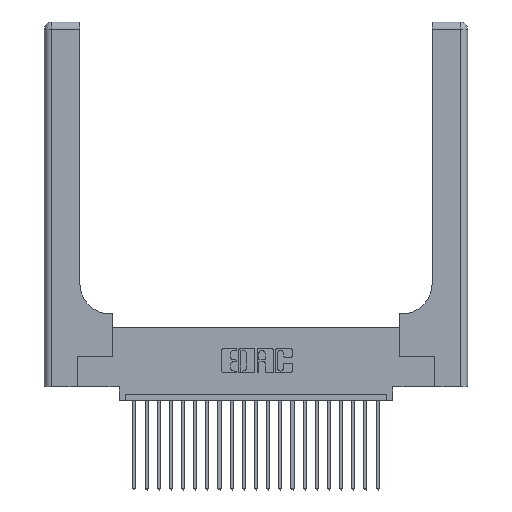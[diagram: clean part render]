
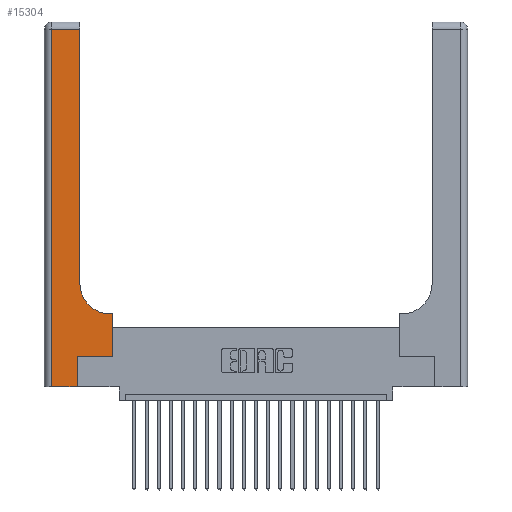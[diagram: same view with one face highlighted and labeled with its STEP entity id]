
A CAD part, top view. The second image highlights one B-rep face of the part: STEP entity #15304.
In plain terms, the highlighted planar face has unit normal (0, 0, 1).
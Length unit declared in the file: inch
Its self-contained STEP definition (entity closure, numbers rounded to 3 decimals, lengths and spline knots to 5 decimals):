
#93 = EDGE_CURVE ( 'NONE', #22028, #8500, #17135, .T. ) ;
#555 = VERTEX_POINT ( 'NONE', #14557 ) ;
#794 = DIRECTION ( 'NONE',  ( 1., 0., 0. ) ) ;
#958 = EDGE_CURVE ( 'NONE', #9788, #2808, #7204, .T. ) ;
#1011 = DIRECTION ( 'NONE',  ( -1., 0., 0. ) ) ;
#2621 = CARTESIAN_POINT ( 'NONE',  ( 0.2915, 3., 0.37 ) ) ;
#2646 = CARTESIAN_POINT ( 'NONE',  ( 0.269, 0., 0.37 ) ) ;
#2687 = EDGE_CURVE ( 'NONE', #6200, #15334, #2757, .T. ) ;
#2757 = LINE ( 'NONE', #19590, #21880 ) ;
#2808 = VERTEX_POINT ( 'NONE', #17730 ) ;
#2962 = LINE ( 'NONE', #18413, #11692 ) ;
#3296 = EDGE_CURVE ( 'NONE', #3470, #6200, #6463, .T. ) ;
#3470 = VERTEX_POINT ( 'NONE', #16917 ) ;
#3796 = EDGE_CURVE ( 'NONE', #8500, #555, #2962, .T. ) ;
#4652 = CARTESIAN_POINT ( 'NONE',  ( 0., 3., 0.37 ) ) ;
#4684 = DIRECTION ( 'NONE',  ( 0., 1., 0. ) ) ;
#4920 = LINE ( 'NONE', #6509, #10421 ) ;
#5051 = DIRECTION ( 'NONE',  ( 0., 1., 0. ) ) ;
#5177 = DIRECTION ( 'NONE',  ( 1., 0., 0. ) ) ;
#5511 = ORIENTED_EDGE ( 'NONE', *, *, #3296, .T. ) ;
#6200 = VERTEX_POINT ( 'NONE', #8472 ) ;
#6463 = LINE ( 'NONE', #14216, #7358 ) ;
#6509 = CARTESIAN_POINT ( 'NONE',  ( 0., 2.94, 0.37 ) ) ;
#6706 = CARTESIAN_POINT ( 'NONE',  ( 0.269, 0.25, 0.37 ) ) ;
#7204 = LINE ( 'NONE', #2621, #10124 ) ;
#7358 = VECTOR ( 'NONE', #5051, 39.37008 ) ;
#8363 = CARTESIAN_POINT ( 'NONE',  ( 0.5415, 0.6, 0.37 ) ) ;
#8472 = CARTESIAN_POINT ( 'NONE',  ( 0.5585, 0.6, 0.37 ) ) ;
#8500 = VERTEX_POINT ( 'NONE', #18981 ) ;
#9495 = CARTESIAN_POINT ( 'NONE',  ( 0.06, 2.94, 0.37 ) ) ;
#9610 = LINE ( 'NONE', #2646, #19750 ) ;
#9763 = ORIENTED_EDGE ( 'NONE', *, *, #3796, .T. ) ;
#9788 = VERTEX_POINT ( 'NONE', #20471 ) ;
#10089 = ORIENTED_EDGE ( 'NONE', *, *, #958, .T. ) ;
#10124 = VECTOR ( 'NONE', #21164, 39.37008 ) ;
#10263 = CARTESIAN_POINT ( 'NONE',  ( 0.06, 3., 0.37 ) ) ;
#10346 = DIRECTION ( 'NONE',  ( 0., -1., 0. ) ) ;
#10421 = VECTOR ( 'NONE', #1011, 39.37008 ) ;
#11050 = EDGE_CURVE ( 'NONE', #15334, #9788, #11296, .T. ) ;
#11296 = CIRCLE ( 'NONE', #23469, 0.25 ) ;
#11692 = VECTOR ( 'NONE', #15731, 39.37008 ) ;
#11892 = DIRECTION ( 'NONE',  ( 0., 0., -1. ) ) ;
#11923 = FACE_OUTER_BOUND ( 'NONE', #21212, .T. ) ;
#12024 = DIRECTION ( 'NONE',  ( -1., 0., 0. ) ) ;
#12341 = VERTEX_POINT ( 'NONE', #6706 ) ;
#12382 = ORIENTED_EDGE ( 'NONE', *, *, #16177, .T. ) ;
#13208 = EDGE_CURVE ( 'NONE', #12341, #3470, #19015, .T. ) ;
#13947 = ORIENTED_EDGE ( 'NONE', *, *, #93, .T. ) ;
#14211 = DIRECTION ( 'NONE',  ( 0., 0., -1. ) ) ;
#14216 = CARTESIAN_POINT ( 'NONE',  ( 0.5585, 0.25, 0.37 ) ) ;
#14430 = ORIENTED_EDGE ( 'NONE', *, *, #11050, .T. ) ;
#14502 = DIRECTION ( 'NONE',  ( -1., 0., 0. ) ) ;
#14557 = CARTESIAN_POINT ( 'NONE',  ( 0.269, 0., 0.37 ) ) ;
#15087 = EDGE_CURVE ( 'NONE', #555, #12341, #9610, .T. ) ;
#15304 = ADVANCED_FACE ( 'NONE', ( #11923 ), #23410, .F. ) ;
#15334 = VERTEX_POINT ( 'NONE', #8363 ) ;
#15379 = ORIENTED_EDGE ( 'NONE', *, *, #13208, .T. ) ;
#15731 = DIRECTION ( 'NONE',  ( 1., 0., 0. ) ) ;
#16177 = EDGE_CURVE ( 'NONE', #2808, #22028, #4920, .T. ) ;
#16917 = CARTESIAN_POINT ( 'NONE',  ( 0.5585, 0.25, 0.37 ) ) ;
#16989 = ORIENTED_EDGE ( 'NONE', *, *, #15087, .T. ) ;
#16991 = VECTOR ( 'NONE', #5177, 39.37008 ) ;
#17135 = LINE ( 'NONE', #10263, #23457 ) ;
#17730 = CARTESIAN_POINT ( 'NONE',  ( 0.2915, 2.94, 0.37 ) ) ;
#18413 = CARTESIAN_POINT ( 'NONE',  ( 0., 0., 0.37 ) ) ;
#18981 = CARTESIAN_POINT ( 'NONE',  ( 0.06, 0., 0.37 ) ) ;
#19015 = LINE ( 'NONE', #23703, #16991 ) ;
#19214 = ORIENTED_EDGE ( 'NONE', *, *, #2687, .T. ) ;
#19549 = CARTESIAN_POINT ( 'NONE',  ( 0.5415, 0.85, 0.37 ) ) ;
#19590 = CARTESIAN_POINT ( 'NONE',  ( 0.2915, 0.6, 0.37 ) ) ;
#19750 = VECTOR ( 'NONE', #4684, 39.37008 ) ;
#20471 = CARTESIAN_POINT ( 'NONE',  ( 0.2915, 0.85, 0.37 ) ) ;
#21164 = DIRECTION ( 'NONE',  ( 0., 1., 0. ) ) ;
#21212 = EDGE_LOOP ( 'NONE', ( #10089, #12382, #13947, #9763, #16989, #15379, #5511, #19214, #14430 ) ) ;
#21880 = VECTOR ( 'NONE', #14502, 39.37008 ) ;
#22028 = VERTEX_POINT ( 'NONE', #9495 ) ;
#23410 = PLANE ( 'NONE',  #23827 ) ;
#23457 = VECTOR ( 'NONE', #10346, 39.37008 ) ;
#23469 = AXIS2_PLACEMENT_3D ( 'NONE', #19549, #11892, #794 ) ;
#23703 = CARTESIAN_POINT ( 'NONE',  ( 0.269, 0.25, 0.37 ) ) ;
#23827 = AXIS2_PLACEMENT_3D ( 'NONE', #4652, #14211, #12024 ) ;
